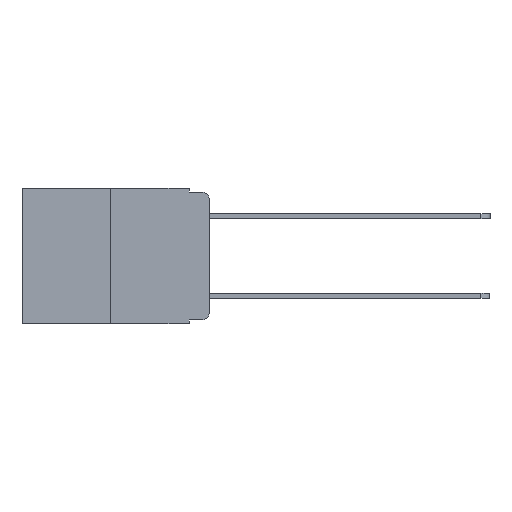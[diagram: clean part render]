
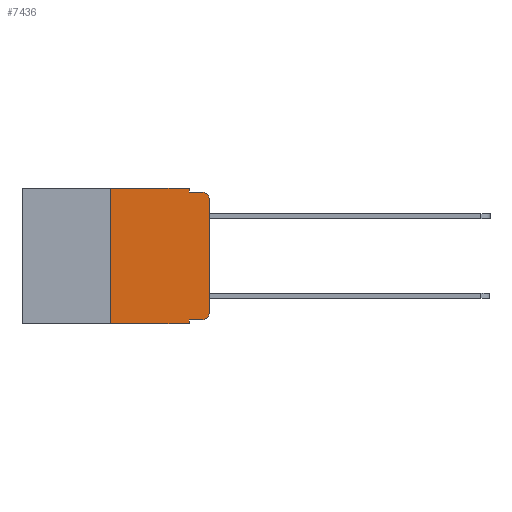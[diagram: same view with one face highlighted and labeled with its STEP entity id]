
A CAD part, left-side view. The second image highlights one B-rep face of the part: STEP entity #7436.
In plain terms, the highlighted planar face has unit normal (-1, 0, 0).
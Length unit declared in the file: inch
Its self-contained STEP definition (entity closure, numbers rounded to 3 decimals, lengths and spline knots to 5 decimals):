
#112 = LINE ( 'NONE', #1262, #4556 ) ;
#119 = CARTESIAN_POINT ( 'NONE',  ( 0., 0.473, 0. ) ) ;
#888 = DIRECTION ( 'NONE',  ( 0., 0., -1. ) ) ;
#934 = CARTESIAN_POINT ( 'NONE',  ( 0., 0.051, -0.01 ) ) ;
#1118 = DIRECTION ( 'NONE',  ( 0., -1., 0. ) ) ;
#1225 = CARTESIAN_POINT ( 'NONE',  ( 0., 0., 0. ) ) ;
#1262 = CARTESIAN_POINT ( 'NONE',  ( 0., 0.051, -0.01 ) ) ;
#1301 = DIRECTION ( 'NONE',  ( 0., 0., -1. ) ) ;
#1583 = FACE_OUTER_BOUND ( 'NONE', #9590, .T. ) ;
#2086 = VECTOR ( 'NONE', #9377, 39.37008 ) ;
#2112 = VECTOR ( 'NONE', #1118, 39.37008 ) ;
#2185 = DIRECTION ( 'NONE',  ( 0., 0., 1. ) ) ;
#2225 = DIRECTION ( 'NONE',  ( -1., 0., 0. ) ) ;
#2270 = CARTESIAN_POINT ( 'NONE',  ( 0., 0.051, 0. ) ) ;
#2307 = CARTESIAN_POINT ( 'NONE',  ( 0., 0.02, -0.313 ) ) ;
#2386 = LINE ( 'NONE', #10099, #11022 ) ;
#2703 = VECTOR ( 'NONE', #2185, 39.37008 ) ;
#2828 = VERTEX_POINT ( 'NONE', #11047 ) ;
#2859 = VERTEX_POINT ( 'NONE', #9460 ) ;
#2864 = ORIENTED_EDGE ( 'NONE', *, *, #10623, .T. ) ;
#3204 = DIRECTION ( 'NONE',  ( 0., 0., 1. ) ) ;
#3250 = DIRECTION ( 'NONE',  ( 0., 0., -1. ) ) ;
#3565 = VERTEX_POINT ( 'NONE', #4541 ) ;
#3711 = ORIENTED_EDGE ( 'NONE', *, *, #11030, .T. ) ;
#4009 = VERTEX_POINT ( 'NONE', #9240 ) ;
#4267 = LINE ( 'NONE', #5041, #10768 ) ;
#4302 = ORIENTED_EDGE ( 'NONE', *, *, #11149, .T. ) ;
#4541 = CARTESIAN_POINT ( 'NONE',  ( 0., 0.051, -0.333 ) ) ;
#4556 = VECTOR ( 'NONE', #10880, 39.37008 ) ;
#4797 = VERTEX_POINT ( 'NONE', #7964 ) ;
#5041 = CARTESIAN_POINT ( 'NONE',  ( 0., 0.051, -0.333 ) ) ;
#5130 = LINE ( 'NONE', #1225, #2703 ) ;
#5441 = LINE ( 'NONE', #6900, #6763 ) ;
#5464 = ORIENTED_EDGE ( 'NONE', *, *, #11088, .F. ) ;
#5703 = VERTEX_POINT ( 'NONE', #10016 ) ;
#5771 = ORIENTED_EDGE ( 'NONE', *, *, #11104, .F. ) ;
#5864 = AXIS2_PLACEMENT_3D ( 'NONE', #9758, #6535, #888 ) ;
#6029 = DIRECTION ( 'NONE',  ( 0., -1., 0. ) ) ;
#6384 = ORIENTED_EDGE ( 'NONE', *, *, #10065, .F. ) ;
#6497 = VERTEX_POINT ( 'NONE', #934 ) ;
#6535 = DIRECTION ( 'NONE',  ( 1., 0., 0. ) ) ;
#6763 = VECTOR ( 'NONE', #3204, 39.37008 ) ;
#6772 = VECTOR ( 'NONE', #7347, 39.37008 ) ;
#6825 = CARTESIAN_POINT ( 'NONE',  ( 0., 0.02, -0.01 ) ) ;
#6855 = VERTEX_POINT ( 'NONE', #9784 ) ;
#6900 = CARTESIAN_POINT ( 'NONE',  ( 0., 0.25, 0. ) ) ;
#6918 = ORIENTED_EDGE ( 'NONE', *, *, #11120, .F. ) ;
#7037 = CIRCLE ( 'NONE', #11344, 0.02 ) ;
#7060 = ORIENTED_EDGE ( 'NONE', *, *, #11071, .T. ) ;
#7347 = DIRECTION ( 'NONE',  ( 0., -1., 0. ) ) ;
#7436 = ADVANCED_FACE ( 'NONE', ( #1583 ), #8208, .F. ) ;
#7738 = CARTESIAN_POINT ( 'NONE',  ( 0., 0.02, -0.03 ) ) ;
#7923 = CARTESIAN_POINT ( 'NONE',  ( 0., 0., -0.313 ) ) ;
#7964 = CARTESIAN_POINT ( 'NONE',  ( 0., 0.25, 0. ) ) ;
#8208 = PLANE ( 'NONE',  #5864 ) ;
#8552 = DIRECTION ( 'NONE',  ( 0., 0., -1. ) ) ;
#8628 = DIRECTION ( 'NONE',  ( -1., 0., 0. ) ) ;
#8759 = ORIENTED_EDGE ( 'NONE', *, *, #11135, .T. ) ;
#8984 = LINE ( 'NONE', #2270, #2086 ) ;
#9240 = CARTESIAN_POINT ( 'NONE',  ( 0., 0.25, -0.343 ) ) ;
#9377 = DIRECTION ( 'NONE',  ( 0., 0., -1. ) ) ;
#9454 = CIRCLE ( 'NONE', #10826, 0.02 ) ;
#9460 = CARTESIAN_POINT ( 'NONE',  ( 0., 0., -0.03 ) ) ;
#9550 = VERTEX_POINT ( 'NONE', #7923 ) ;
#9590 = EDGE_LOOP ( 'NONE', ( #3711, #7060, #5464, #5771, #6384, #6918, #2864, #10315, #8759, #4302 ) ) ;
#9758 = CARTESIAN_POINT ( 'NONE',  ( 0., 0.473, 0. ) ) ;
#9784 = CARTESIAN_POINT ( 'NONE',  ( 0., 0.02, -0.333 ) ) ;
#10016 = CARTESIAN_POINT ( 'NONE',  ( 0., 0.051, -0.343 ) ) ;
#10065 = EDGE_CURVE ( 'NONE', #4797, #2828, #11043, .T. ) ;
#10099 = CARTESIAN_POINT ( 'NONE',  ( 0., 0.051, 0. ) ) ;
#10315 = ORIENTED_EDGE ( 'NONE', *, *, #11131, .F. ) ;
#10623 = EDGE_CURVE ( 'NONE', #4009, #5703, #11268, .T. ) ;
#10768 = VECTOR ( 'NONE', #6029, 39.37008 ) ;
#10826 = AXIS2_PLACEMENT_3D ( 'NONE', #7738, #2225, #8552 ) ;
#10880 = DIRECTION ( 'NONE',  ( 0., -1., 0. ) ) ;
#11022 = VECTOR ( 'NONE', #1301, 39.37008 ) ;
#11028 = VERTEX_POINT ( 'NONE', #6825 ) ;
#11030 = EDGE_CURVE ( 'NONE', #9550, #2859, #5130, .T. ) ;
#11043 = LINE ( 'NONE', #119, #2112 ) ;
#11047 = CARTESIAN_POINT ( 'NONE',  ( 0., 0.051, 0. ) ) ;
#11071 = EDGE_CURVE ( 'NONE', #2859, #11028, #9454, .T. ) ;
#11088 = EDGE_CURVE ( 'NONE', #6497, #11028, #112, .T. ) ;
#11104 = EDGE_CURVE ( 'NONE', #2828, #6497, #2386, .T. ) ;
#11120 = EDGE_CURVE ( 'NONE', #4009, #4797, #5441, .T. ) ;
#11131 = EDGE_CURVE ( 'NONE', #3565, #5703, #8984, .T. ) ;
#11135 = EDGE_CURVE ( 'NONE', #3565, #6855, #4267, .T. ) ;
#11149 = EDGE_CURVE ( 'NONE', #6855, #9550, #7037, .T. ) ;
#11265 = CARTESIAN_POINT ( 'NONE',  ( 0., 0.473, -0.343 ) ) ;
#11268 = LINE ( 'NONE', #11265, #6772 ) ;
#11344 = AXIS2_PLACEMENT_3D ( 'NONE', #2307, #8628, #3250 ) ;
